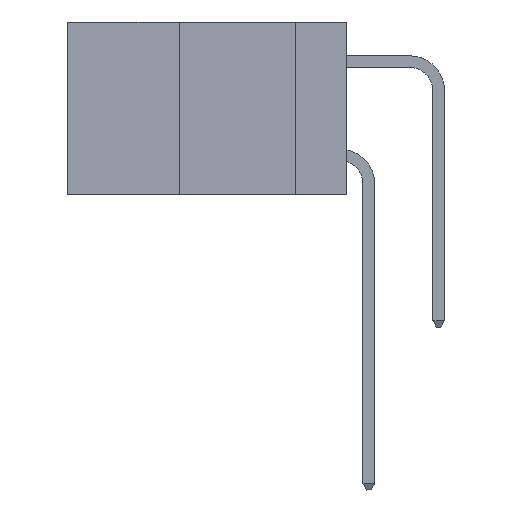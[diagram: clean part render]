
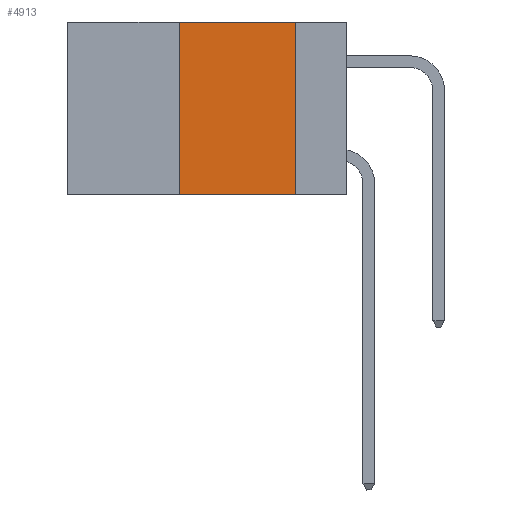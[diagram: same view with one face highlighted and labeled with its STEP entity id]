
A CAD part, left-side view. The second image highlights one B-rep face of the part: STEP entity #4913.
In plain terms, the highlighted planar face has unit normal (-1, 0, 0).
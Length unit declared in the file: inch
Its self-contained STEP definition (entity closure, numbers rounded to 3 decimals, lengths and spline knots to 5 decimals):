
#1754 = LINE ( 'NONE', #12130, #38946 ) ;
#3356 = VECTOR ( 'NONE', #33682, 39.37008 ) ;
#4913 = ADVANCED_FACE ( 'NONE', ( #32498 ), #13187, .F. ) ;
#4962 = DIRECTION ( 'NONE',  ( 0., 0., -1. ) ) ;
#5753 = VERTEX_POINT ( 'NONE', #34858 ) ;
#6067 = CARTESIAN_POINT ( 'NONE',  ( 0., 0.6, 0. ) ) ;
#6245 = EDGE_CURVE ( 'NONE', #16353, #32756, #42529, .T. ) ;
#12130 = CARTESIAN_POINT ( 'NONE',  ( 0., 0.11, 0. ) ) ;
#12808 = LINE ( 'NONE', #19903, #3356 ) ;
#13187 = PLANE ( 'NONE',  #20264 ) ;
#13226 = CARTESIAN_POINT ( 'NONE',  ( 0., 0.36, 0. ) ) ;
#13237 = VECTOR ( 'NONE', #17282, 39.37008 ) ;
#14342 = LINE ( 'NONE', #24489, #13237 ) ;
#16353 = VERTEX_POINT ( 'NONE', #32048 ) ;
#16631 = DIRECTION ( 'NONE',  ( 0., 0., 1. ) ) ;
#17148 = VECTOR ( 'NONE', #16631, 39.37008 ) ;
#17282 = DIRECTION ( 'NONE',  ( 0., -1., 0. ) ) ;
#18113 = ORIENTED_EDGE ( 'NONE', *, *, #6245, .F. ) ;
#19903 = CARTESIAN_POINT ( 'NONE',  ( 0., 0.6, -0.37 ) ) ;
#20264 = AXIS2_PLACEMENT_3D ( 'NONE', #6067, #44338, #23810 ) ;
#21476 = VERTEX_POINT ( 'NONE', #30855 ) ;
#22989 = ORIENTED_EDGE ( 'NONE', *, *, #27308, .F. ) ;
#23810 = DIRECTION ( 'NONE',  ( 0., 0., -1. ) ) ;
#24489 = CARTESIAN_POINT ( 'NONE',  ( 0., 0.6, 0. ) ) ;
#25170 = EDGE_CURVE ( 'NONE', #16353, #5753, #12808, .T. ) ;
#27308 = EDGE_CURVE ( 'NONE', #32756, #21476, #14342, .T. ) ;
#30855 = CARTESIAN_POINT ( 'NONE',  ( 0., 0.11, 0. ) ) ;
#32048 = CARTESIAN_POINT ( 'NONE',  ( 0., 0.36, -0.37 ) ) ;
#32171 = ORIENTED_EDGE ( 'NONE', *, *, #25170, .T. ) ;
#32498 = FACE_OUTER_BOUND ( 'NONE', #39919, .T. ) ;
#32756 = VERTEX_POINT ( 'NONE', #13226 ) ;
#33682 = DIRECTION ( 'NONE',  ( 0., -1., 0. ) ) ;
#34858 = CARTESIAN_POINT ( 'NONE',  ( 0., 0.11, -0.37 ) ) ;
#37375 = CARTESIAN_POINT ( 'NONE',  ( 0., 0.36, 0. ) ) ;
#38025 = ORIENTED_EDGE ( 'NONE', *, *, #38944, .F. ) ;
#38944 = EDGE_CURVE ( 'NONE', #21476, #5753, #1754, .T. ) ;
#38946 = VECTOR ( 'NONE', #4962, 39.37008 ) ;
#39919 = EDGE_LOOP ( 'NONE', ( #38025, #22989, #18113, #32171 ) ) ;
#42529 = LINE ( 'NONE', #37375, #17148 ) ;
#44338 = DIRECTION ( 'NONE',  ( 1., 0., 0. ) ) ;
